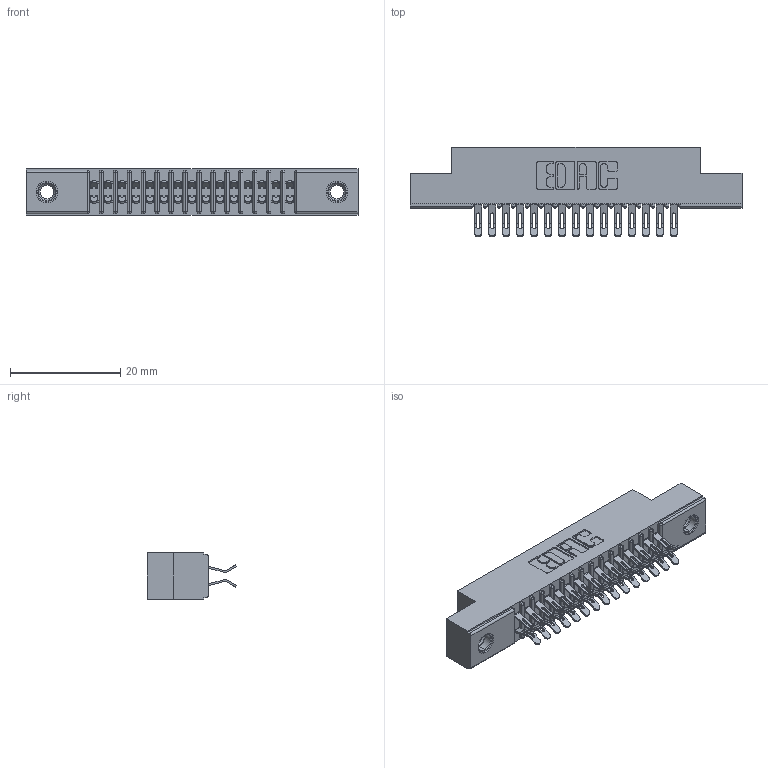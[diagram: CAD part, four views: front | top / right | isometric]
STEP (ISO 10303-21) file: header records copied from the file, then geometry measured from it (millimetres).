
FILE_DESCRIPTION (( 'STEP AP203' ), '1' );
FILE_NAME ('391-030-555-207.STEP', '2018-08-08T21:41:08', ( '' ), ( '' ), 'SwSTEP 2.0', 'SolidWorks 2016', '' );
FILE_SCHEMA (( 'CONFIG_CONTROL_DESIGN' ));
Length unit declared in the file: inch
Products named in the file (4): 341-292-001_341-292-155; 345-250-001_345-250-005-103; 391-030-555-207; 341 Part_.156 (3.96) Dia Mounting Holes
Assembly tree (33 placements, depth 2):
  391-030-555-207
    341 Part_.156 (3.96) Dia Mounting Holes
    341-292-001_341-292-155  x30
    345-250-001_345-250-005-103  x2
Bounding box: 60.33 x 16.31 x 8.38 mm (x, y, z)
Volume: 3478.1 mm3; surface area: 7085.6 mm2
Topology: 33 solids, 33 shells, 2516 faces, 7457 edges, 4850 vertices
Faces by surface type: plane 1360, cylinder 1080, sphere 32, torus 32, cone 12
Entity records: 23405 total; most frequent: CARTESIAN_POINT 3890, ORIENTED_EDGE 3846, DIRECTION 3795, EDGE_CURVE 1923, LINE 1505, VECTOR 1505, VERTEX_POINT 1224, AXIS2_PLACEMENT_3D 1145
